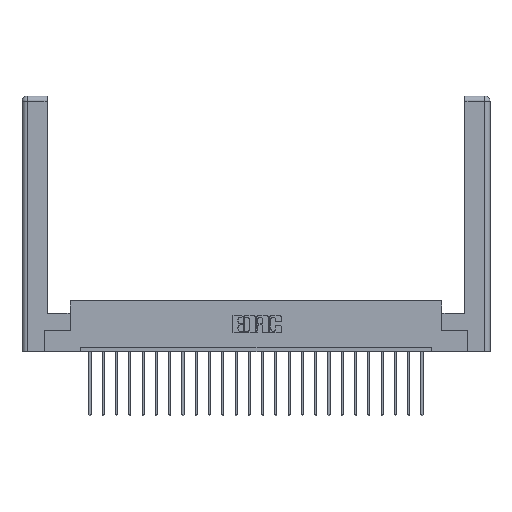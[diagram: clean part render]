
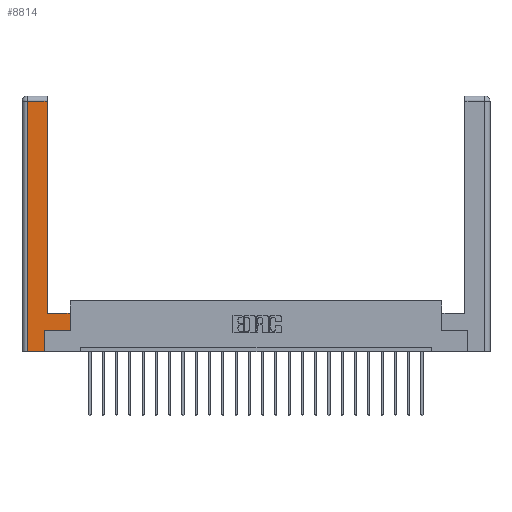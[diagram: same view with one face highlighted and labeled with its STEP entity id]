
A CAD part, top view. The second image highlights one B-rep face of the part: STEP entity #8814.
In plain terms, the highlighted planar face has unit normal (0, 0, 1).
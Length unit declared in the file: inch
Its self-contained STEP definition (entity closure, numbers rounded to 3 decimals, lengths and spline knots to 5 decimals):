
#418 = LINE ( 'NONE', #22323, #1007 ) ;
#567 = EDGE_CURVE ( 'NONE', #16746, #2839, #4872, .T. ) ;
#1007 = VECTOR ( 'NONE', #11018, 39.37008 ) ;
#1073 = VERTEX_POINT ( 'NONE', #4198 ) ;
#1439 = CARTESIAN_POINT ( 'NONE',  ( 0.565, 0.245, 0. ) ) ;
#1661 = VERTEX_POINT ( 'NONE', #7004 ) ;
#2612 = CARTESIAN_POINT ( 'NONE',  ( 0.265, 0.245, 0. ) ) ;
#2725 = VECTOR ( 'NONE', #10374, 39.37008 ) ;
#2839 = VERTEX_POINT ( 'NONE', #20482 ) ;
#3023 = VECTOR ( 'NONE', #8061, 39.37008 ) ;
#3185 = EDGE_CURVE ( 'NONE', #2839, #1073, #23026, .T. ) ;
#3855 = CARTESIAN_POINT ( 'NONE',  ( 0.0615, 0., 0. ) ) ;
#4195 = EDGE_CURVE ( 'NONE', #7822, #18874, #14170, .T. ) ;
#4198 = CARTESIAN_POINT ( 'NONE',  ( 0.295, 2.94, 0. ) ) ;
#4281 = VECTOR ( 'NONE', #22658, 39.37008 ) ;
#4349 = CARTESIAN_POINT ( 'NONE',  ( 0.265, 0., 0. ) ) ;
#4461 = ORIENTED_EDGE ( 'NONE', *, *, #23946, .T. ) ;
#4872 = LINE ( 'NONE', #22531, #11239 ) ;
#4951 = FACE_OUTER_BOUND ( 'NONE', #11847, .T. ) ;
#5590 = DIRECTION ( 'NONE',  ( -1., 0., 0. ) ) ;
#5682 = EDGE_CURVE ( 'NONE', #1661, #18016, #11984, .T. ) ;
#6384 = CARTESIAN_POINT ( 'NONE',  ( 0.565, 0.45, 0. ) ) ;
#6883 = DIRECTION ( 'NONE',  ( 1., 0., 0. ) ) ;
#6953 = CARTESIAN_POINT ( 'NONE',  ( 0.265, 0.245, 0. ) ) ;
#7004 = CARTESIAN_POINT ( 'NONE',  ( 0.265, 0., 0. ) ) ;
#7583 = VECTOR ( 'NONE', #13540, 39.37008 ) ;
#7822 = VERTEX_POINT ( 'NONE', #21839 ) ;
#8061 = DIRECTION ( 'NONE',  ( 0., 1., 0. ) ) ;
#8170 = CARTESIAN_POINT ( 'NONE',  ( 0., 0., 0. ) ) ;
#8814 = ADVANCED_FACE ( 'NONE', ( #4951 ), #22818, .F. ) ;
#9277 = ORIENTED_EDGE ( 'NONE', *, *, #16618, .T. ) ;
#9340 = VECTOR ( 'NONE', #6883, 39.37008 ) ;
#9785 = ORIENTED_EDGE ( 'NONE', *, *, #18725, .T. ) ;
#10374 = DIRECTION ( 'NONE',  ( 0., 1., 0. ) ) ;
#10444 = AXIS2_PLACEMENT_3D ( 'NONE', #8170, #13538, #19125 ) ;
#10445 = CARTESIAN_POINT ( 'NONE',  ( 0.295, 3., 0. ) ) ;
#10588 = ORIENTED_EDGE ( 'NONE', *, *, #4195, .T. ) ;
#11018 = DIRECTION ( 'NONE',  ( -1., 0., 0. ) ) ;
#11239 = VECTOR ( 'NONE', #5590, 39.37008 ) ;
#11510 = CARTESIAN_POINT ( 'NONE',  ( 0.565, 0.45, 0. ) ) ;
#11825 = ORIENTED_EDGE ( 'NONE', *, *, #567, .T. ) ;
#11847 = EDGE_LOOP ( 'NONE', ( #18515, #9277, #10588, #20289, #18053, #9785, #4461, #11825 ) ) ;
#11984 = LINE ( 'NONE', #2612, #3023 ) ;
#13538 = DIRECTION ( 'NONE',  ( 0., 0., -1. ) ) ;
#13540 = DIRECTION ( 'NONE',  ( 0., 1., 0. ) ) ;
#14170 = LINE ( 'NONE', #3855, #4281 ) ;
#16569 = LINE ( 'NONE', #6384, #7583 ) ;
#16610 = CARTESIAN_POINT ( 'NONE',  ( 0.565, 0.245, 0. ) ) ;
#16618 = EDGE_CURVE ( 'NONE', #1073, #7822, #418, .T. ) ;
#16746 = VERTEX_POINT ( 'NONE', #11510 ) ;
#17881 = VECTOR ( 'NONE', #23105, 39.37008 ) ;
#18016 = VERTEX_POINT ( 'NONE', #6953 ) ;
#18053 = ORIENTED_EDGE ( 'NONE', *, *, #5682, .T. ) ;
#18515 = ORIENTED_EDGE ( 'NONE', *, *, #3185, .T. ) ;
#18725 = EDGE_CURVE ( 'NONE', #18016, #18903, #21529, .T. ) ;
#18874 = VERTEX_POINT ( 'NONE', #23886 ) ;
#18903 = VERTEX_POINT ( 'NONE', #16610 ) ;
#19125 = DIRECTION ( 'NONE',  ( -1., 0., 0. ) ) ;
#20289 = ORIENTED_EDGE ( 'NONE', *, *, #22012, .T. ) ;
#20482 = CARTESIAN_POINT ( 'NONE',  ( 0.295, 0.45, 0. ) ) ;
#21529 = LINE ( 'NONE', #1439, #9340 ) ;
#21839 = CARTESIAN_POINT ( 'NONE',  ( 0.0615, 2.94, 0. ) ) ;
#22012 = EDGE_CURVE ( 'NONE', #18874, #1661, #22819, .T. ) ;
#22323 = CARTESIAN_POINT ( 'NONE',  ( 0.0615, 2.94, 0. ) ) ;
#22531 = CARTESIAN_POINT ( 'NONE',  ( 0.295, 0.45, 0. ) ) ;
#22658 = DIRECTION ( 'NONE',  ( 0., -1., 0. ) ) ;
#22818 = PLANE ( 'NONE',  #10444 ) ;
#22819 = LINE ( 'NONE', #4349, #17881 ) ;
#23026 = LINE ( 'NONE', #10445, #2725 ) ;
#23105 = DIRECTION ( 'NONE',  ( 1., 0., 0. ) ) ;
#23886 = CARTESIAN_POINT ( 'NONE',  ( 0.0615, 0., 0. ) ) ;
#23946 = EDGE_CURVE ( 'NONE', #18903, #16746, #16569, .T. ) ;
